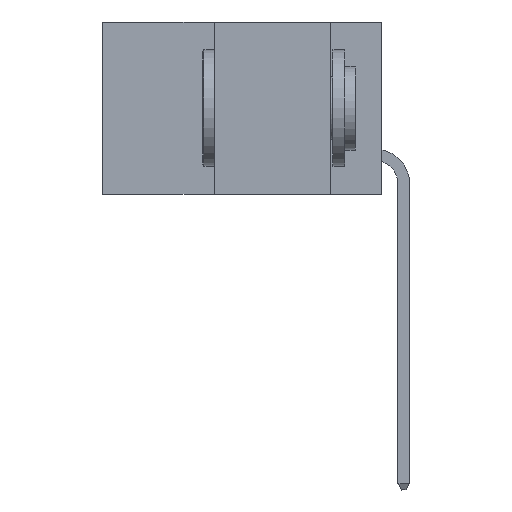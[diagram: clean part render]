
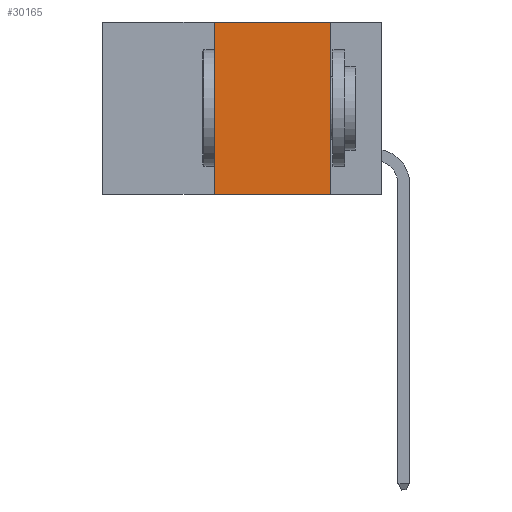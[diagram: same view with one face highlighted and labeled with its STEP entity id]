
A CAD part, left-side view. The second image highlights one B-rep face of the part: STEP entity #30165.
In plain terms, the highlighted planar face has unit normal (-1, 0, 0).
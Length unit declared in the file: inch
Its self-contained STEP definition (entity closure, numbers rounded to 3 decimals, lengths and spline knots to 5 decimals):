
#175 = EDGE_CURVE ( 'NONE', #45085, #27727, #20004, .T. ) ;
#1163 = DIRECTION ( 'NONE',  ( 0., 0., 1. ) ) ;
#1550 = CARTESIAN_POINT ( 'NONE',  ( 0., 0.11, -0.37 ) ) ;
#3199 = VECTOR ( 'NONE', #5248, 39.37008 ) ;
#5248 = DIRECTION ( 'NONE',  ( 0., 0., -1. ) ) ;
#7031 = VERTEX_POINT ( 'NONE', #31306 ) ;
#7043 = EDGE_LOOP ( 'NONE', ( #11412, #7434, #16251, #39493 ) ) ;
#7434 = ORIENTED_EDGE ( 'NONE', *, *, #35679, .F. ) ;
#9078 = VECTOR ( 'NONE', #26340, 39.37008 ) ;
#11412 = ORIENTED_EDGE ( 'NONE', *, *, #39314, .F. ) ;
#12341 = CARTESIAN_POINT ( 'NONE',  ( 0., 0.6, -0.37 ) ) ;
#13394 = LINE ( 'NONE', #40498, #41322 ) ;
#15734 = DIRECTION ( 'NONE',  ( 0., -1., 0. ) ) ;
#15843 = CARTESIAN_POINT ( 'NONE',  ( 0., 0.11, 0. ) ) ;
#16251 = ORIENTED_EDGE ( 'NONE', *, *, #30074, .F. ) ;
#17478 = CARTESIAN_POINT ( 'NONE',  ( 0., 0.36, -0.37 ) ) ;
#18015 = FACE_OUTER_BOUND ( 'NONE', #7043, .T. ) ;
#20004 = LINE ( 'NONE', #12341, #29678 ) ;
#24443 = LINE ( 'NONE', #15843, #3199 ) ;
#26187 = DIRECTION ( 'NONE',  ( 0., 0., -1. ) ) ;
#26340 = DIRECTION ( 'NONE',  ( 0., -1., 0. ) ) ;
#27727 = VERTEX_POINT ( 'NONE', #1550 ) ;
#29678 = VECTOR ( 'NONE', #15734, 39.37008 ) ;
#30074 = EDGE_CURVE ( 'NONE', #45085, #7031, #13394, .T. ) ;
#30165 = ADVANCED_FACE ( 'NONE', ( #18015 ), #44786, .F. ) ;
#31306 = CARTESIAN_POINT ( 'NONE',  ( 0., 0.36, 0. ) ) ;
#33948 = CARTESIAN_POINT ( 'NONE',  ( 0., 0.6, 0. ) ) ;
#35679 = EDGE_CURVE ( 'NONE', #7031, #38822, #41092, .T. ) ;
#38822 = VERTEX_POINT ( 'NONE', #39593 ) ;
#39314 = EDGE_CURVE ( 'NONE', #38822, #27727, #24443, .T. ) ;
#39493 = ORIENTED_EDGE ( 'NONE', *, *, #175, .T. ) ;
#39593 = CARTESIAN_POINT ( 'NONE',  ( 0., 0.11, 0. ) ) ;
#40483 = DIRECTION ( 'NONE',  ( 1., 0., 0. ) ) ;
#40498 = CARTESIAN_POINT ( 'NONE',  ( 0., 0.36, 0. ) ) ;
#41092 = LINE ( 'NONE', #44647, #9078 ) ;
#41322 = VECTOR ( 'NONE', #1163, 39.37008 ) ;
#43911 = AXIS2_PLACEMENT_3D ( 'NONE', #33948, #40483, #26187 ) ;
#44647 = CARTESIAN_POINT ( 'NONE',  ( 0., 0.6, 0. ) ) ;
#44786 = PLANE ( 'NONE',  #43911 ) ;
#45085 = VERTEX_POINT ( 'NONE', #17478 ) ;
